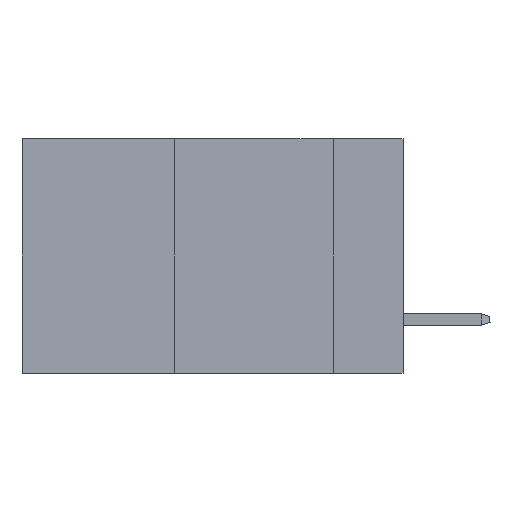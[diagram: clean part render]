
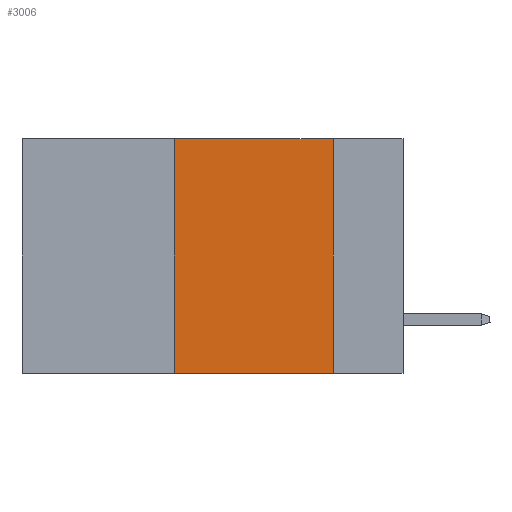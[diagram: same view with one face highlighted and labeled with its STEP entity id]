
A CAD part, left-side view. The second image highlights one B-rep face of the part: STEP entity #3006.
In plain terms, the highlighted planar face has unit normal (-1, 0, 0).
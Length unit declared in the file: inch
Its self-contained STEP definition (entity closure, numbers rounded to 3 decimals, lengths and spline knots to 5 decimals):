
#181 = AXIS2_PLACEMENT_3D ( 'NONE', #8918, #9110, #3265 ) ;
#209 = CARTESIAN_POINT ( 'NONE',  ( 0., 0.11, 0. ) ) ;
#347 = LINE ( 'NONE', #5692, #11275 ) ;
#459 = VERTEX_POINT ( 'NONE', #209 ) ;
#956 = CARTESIAN_POINT ( 'NONE',  ( 0., 0.6, -0.37 ) ) ;
#1391 = EDGE_CURVE ( 'NONE', #459, #4741, #10295, .T. ) ;
#1587 = VERTEX_POINT ( 'NONE', #15093 ) ;
#1882 = CARTESIAN_POINT ( 'NONE',  ( 0., 0.11, 0. ) ) ;
#1886 = EDGE_CURVE ( 'NONE', #16847, #1587, #347, .T. ) ;
#1999 = PLANE ( 'NONE',  #181 ) ;
#2069 = DIRECTION ( 'NONE',  ( 0., 0., -1. ) ) ;
#2245 = EDGE_LOOP ( 'NONE', ( #6430, #2532, #10496, #8444 ) ) ;
#2532 = ORIENTED_EDGE ( 'NONE', *, *, #13231, .F. ) ;
#3006 = ADVANCED_FACE ( 'NONE', ( #15783 ), #1999, .F. ) ;
#3265 = DIRECTION ( 'NONE',  ( 0., 0., -1. ) ) ;
#4741 = VERTEX_POINT ( 'NONE', #6316 ) ;
#5692 = CARTESIAN_POINT ( 'NONE',  ( 0., 0.36, 0. ) ) ;
#6064 = LINE ( 'NONE', #13372, #12595 ) ;
#6316 = CARTESIAN_POINT ( 'NONE',  ( 0., 0.11, -0.37 ) ) ;
#6430 = ORIENTED_EDGE ( 'NONE', *, *, #1391, .F. ) ;
#6845 = VECTOR ( 'NONE', #2069, 39.37008 ) ;
#7782 = LINE ( 'NONE', #956, #8790 ) ;
#8444 = ORIENTED_EDGE ( 'NONE', *, *, #13731, .T. ) ;
#8790 = VECTOR ( 'NONE', #18030, 39.37008 ) ;
#8918 = CARTESIAN_POINT ( 'NONE',  ( 0., 0.6, 0. ) ) ;
#9110 = DIRECTION ( 'NONE',  ( 1., 0., 0. ) ) ;
#10295 = LINE ( 'NONE', #1882, #6845 ) ;
#10496 = ORIENTED_EDGE ( 'NONE', *, *, #1886, .F. ) ;
#11275 = VECTOR ( 'NONE', #12662, 39.37008 ) ;
#12595 = VECTOR ( 'NONE', #15958, 39.37008 ) ;
#12662 = DIRECTION ( 'NONE',  ( 0., 0., 1. ) ) ;
#13231 = EDGE_CURVE ( 'NONE', #1587, #459, #6064, .T. ) ;
#13372 = CARTESIAN_POINT ( 'NONE',  ( 0., 0.6, 0. ) ) ;
#13731 = EDGE_CURVE ( 'NONE', #16847, #4741, #7782, .T. ) ;
#15093 = CARTESIAN_POINT ( 'NONE',  ( 0., 0.36, 0. ) ) ;
#15783 = FACE_OUTER_BOUND ( 'NONE', #2245, .T. ) ;
#15958 = DIRECTION ( 'NONE',  ( 0., -1., 0. ) ) ;
#16716 = CARTESIAN_POINT ( 'NONE',  ( 0., 0.36, -0.37 ) ) ;
#16847 = VERTEX_POINT ( 'NONE', #16716 ) ;
#18030 = DIRECTION ( 'NONE',  ( 0., -1., 0. ) ) ;
